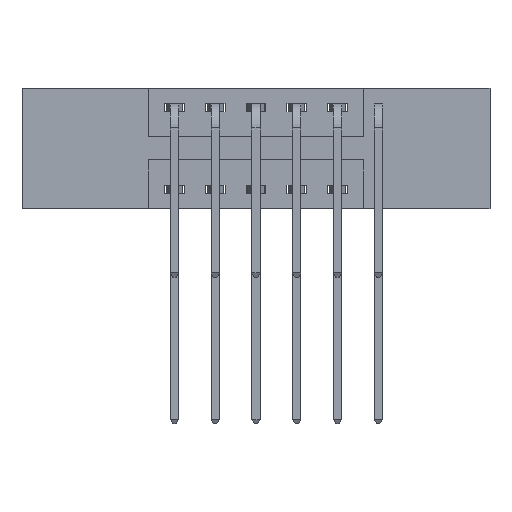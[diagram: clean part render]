
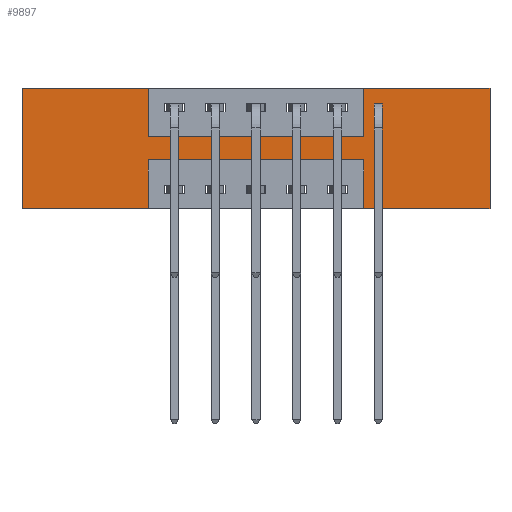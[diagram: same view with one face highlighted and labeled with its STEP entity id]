
A CAD part, front view. The second image highlights one B-rep face of the part: STEP entity #9897.
In plain terms, the highlighted planar face has unit normal (0, -1, 0).
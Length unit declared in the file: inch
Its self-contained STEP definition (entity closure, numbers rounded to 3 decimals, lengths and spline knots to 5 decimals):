
#41 = CARTESIAN_POINT ( 'NONE',  ( 1.435, 0., -0.37 ) ) ;
#46 = CARTESIAN_POINT ( 'NONE',  ( 0., 0., -0.37 ) ) ;
#98 = VECTOR ( 'NONE', #6321, 39.37008 ) ;
#140 = VERTEX_POINT ( 'NONE', #5157 ) ;
#458 = EDGE_CURVE ( 'NONE', #7896, #7610, #5863, .T. ) ;
#606 = CARTESIAN_POINT ( 'NONE',  ( 1.435, 0., 0. ) ) ;
#883 = VERTEX_POINT ( 'NONE', #3703 ) ;
#994 = CARTESIAN_POINT ( 'NONE',  ( 1.435, 0., 0. ) ) ;
#1152 = VERTEX_POINT ( 'NONE', #41 ) ;
#1199 = EDGE_CURVE ( 'NONE', #9735, #4054, #1919, .T. ) ;
#1211 = LINE ( 'NONE', #994, #6348 ) ;
#1308 = DIRECTION ( 'NONE',  ( 0., 0., 1. ) ) ;
#1459 = CARTESIAN_POINT ( 'NONE',  ( 0.3875, 0., -0.37 ) ) ;
#1533 = CARTESIAN_POINT ( 'NONE',  ( 0., 0., 0. ) ) ;
#1675 = VECTOR ( 'NONE', #2664, 39.37008 ) ;
#1687 = VECTOR ( 'NONE', #7762, 39.37008 ) ;
#1724 = EDGE_LOOP ( 'NONE', ( #9180, #6241, #3823, #4499, #4853, #9220, #1844, #4583, #4867, #7285, #4991, #7064 ) ) ;
#1844 = ORIENTED_EDGE ( 'NONE', *, *, #5600, .F. ) ;
#1856 = DIRECTION ( 'NONE',  ( 0., -1., 0. ) ) ;
#1919 = LINE ( 'NONE', #9070, #9211 ) ;
#2128 = LINE ( 'NONE', #1459, #5531 ) ;
#2365 = EDGE_CURVE ( 'NONE', #140, #2655, #6531, .T. ) ;
#2530 = VERTEX_POINT ( 'NONE', #3229 ) ;
#2655 = VERTEX_POINT ( 'NONE', #8426 ) ;
#2664 = DIRECTION ( 'NONE',  ( 0., 0., -1. ) ) ;
#2709 = CARTESIAN_POINT ( 'NONE',  ( 0., 0., 0. ) ) ;
#2813 = LINE ( 'NONE', #6730, #1675 ) ;
#3221 = CARTESIAN_POINT ( 'NONE',  ( 1.0475, 0., 0. ) ) ;
#3229 = CARTESIAN_POINT ( 'NONE',  ( 1.0475, 0., 0. ) ) ;
#3276 = CARTESIAN_POINT ( 'NONE',  ( 0., 0., 0. ) ) ;
#3323 = DIRECTION ( 'NONE',  ( 0., 0., -1. ) ) ;
#3421 = FACE_OUTER_BOUND ( 'NONE', #1724, .T. ) ;
#3545 = DIRECTION ( 'NONE',  ( 0., 0., 1. ) ) ;
#3548 = EDGE_CURVE ( 'NONE', #4054, #8910, #2813, .T. ) ;
#3703 = CARTESIAN_POINT ( 'NONE',  ( 1.0475, 0., -0.37 ) ) ;
#3823 = ORIENTED_EDGE ( 'NONE', *, *, #7267, .F. ) ;
#4054 = VERTEX_POINT ( 'NONE', #9973 ) ;
#4129 = DIRECTION ( 'NONE',  ( -1., 0., 0. ) ) ;
#4168 = DIRECTION ( 'NONE',  ( 0., 0., -1. ) ) ;
#4171 = VERTEX_POINT ( 'NONE', #9597 ) ;
#4249 = AXIS2_PLACEMENT_3D ( 'NONE', #9752, #1856, #3323 ) ;
#4404 = VECTOR ( 'NONE', #3545, 39.37008 ) ;
#4499 = ORIENTED_EDGE ( 'NONE', *, *, #7570, .F. ) ;
#4583 = ORIENTED_EDGE ( 'NONE', *, *, #4963, .F. ) ;
#4853 = ORIENTED_EDGE ( 'NONE', *, *, #9495, .F. ) ;
#4867 = ORIENTED_EDGE ( 'NONE', *, *, #3548, .F. ) ;
#4963 = EDGE_CURVE ( 'NONE', #8910, #4171, #8675, .T. ) ;
#4991 = ORIENTED_EDGE ( 'NONE', *, *, #9981, .F. ) ;
#5035 = LINE ( 'NONE', #8231, #4404 ) ;
#5108 = VECTOR ( 'NONE', #9667, 39.37008 ) ;
#5157 = CARTESIAN_POINT ( 'NONE',  ( 1.0475, 0., -0.22 ) ) ;
#5531 = VECTOR ( 'NONE', #9964, 39.37008 ) ;
#5600 = EDGE_CURVE ( 'NONE', #4171, #2530, #8314, .T. ) ;
#5735 = VECTOR ( 'NONE', #4129, 39.37008 ) ;
#5751 = LINE ( 'NONE', #2709, #7991 ) ;
#5863 = LINE ( 'NONE', #5962, #5108 ) ;
#5962 = CARTESIAN_POINT ( 'NONE',  ( 0., 0., -0.37 ) ) ;
#6241 = ORIENTED_EDGE ( 'NONE', *, *, #2365, .F. ) ;
#6321 = DIRECTION ( 'NONE',  ( -1., 0., 0. ) ) ;
#6348 = VECTOR ( 'NONE', #4168, 39.37008 ) ;
#6393 = EDGE_CURVE ( 'NONE', #2655, #7896, #2128, .T. ) ;
#6531 = LINE ( 'NONE', #9519, #5735 ) ;
#6652 = PLANE ( 'NONE',  #4249 ) ;
#6730 = CARTESIAN_POINT ( 'NONE',  ( 0.3875, 0., 0. ) ) ;
#6998 = VECTOR ( 'NONE', #9552, 39.37008 ) ;
#7064 = ORIENTED_EDGE ( 'NONE', *, *, #458, .F. ) ;
#7090 = LINE ( 'NONE', #46, #98 ) ;
#7267 = EDGE_CURVE ( 'NONE', #883, #140, #5035, .T. ) ;
#7285 = ORIENTED_EDGE ( 'NONE', *, *, #1199, .F. ) ;
#7482 = LINE ( 'NONE', #1533, #9790 ) ;
#7504 = DIRECTION ( 'NONE',  ( 1., 0., 0. ) ) ;
#7570 = EDGE_CURVE ( 'NONE', #1152, #883, #7090, .T. ) ;
#7610 = VERTEX_POINT ( 'NONE', #8118 ) ;
#7674 = EDGE_CURVE ( 'NONE', #2530, #8698, #5751, .T. ) ;
#7762 = DIRECTION ( 'NONE',  ( 1., 0., 0. ) ) ;
#7896 = VERTEX_POINT ( 'NONE', #10062 ) ;
#7910 = CARTESIAN_POINT ( 'NONE',  ( 0.3875, 0., -0.15 ) ) ;
#7991 = VECTOR ( 'NONE', #7504, 39.37008 ) ;
#8118 = CARTESIAN_POINT ( 'NONE',  ( 0., 0., -0.37 ) ) ;
#8231 = CARTESIAN_POINT ( 'NONE',  ( 1.0475, 0., -0.37 ) ) ;
#8314 = LINE ( 'NONE', #3221, #6998 ) ;
#8426 = CARTESIAN_POINT ( 'NONE',  ( 0.3875, 0., -0.22 ) ) ;
#8675 = LINE ( 'NONE', #7910, #1687 ) ;
#8698 = VERTEX_POINT ( 'NONE', #606 ) ;
#8729 = CARTESIAN_POINT ( 'NONE',  ( 0.3875, 0., -0.15 ) ) ;
#8910 = VERTEX_POINT ( 'NONE', #8729 ) ;
#9070 = CARTESIAN_POINT ( 'NONE',  ( 0., 0., 0. ) ) ;
#9180 = ORIENTED_EDGE ( 'NONE', *, *, #6393, .F. ) ;
#9211 = VECTOR ( 'NONE', #9771, 39.37008 ) ;
#9220 = ORIENTED_EDGE ( 'NONE', *, *, #7674, .F. ) ;
#9495 = EDGE_CURVE ( 'NONE', #8698, #1152, #1211, .T. ) ;
#9519 = CARTESIAN_POINT ( 'NONE',  ( 0.3875, 0., -0.22 ) ) ;
#9552 = DIRECTION ( 'NONE',  ( 0., 0., 1. ) ) ;
#9597 = CARTESIAN_POINT ( 'NONE',  ( 1.0475, 0., -0.15 ) ) ;
#9667 = DIRECTION ( 'NONE',  ( -1., 0., 0. ) ) ;
#9735 = VERTEX_POINT ( 'NONE', #3276 ) ;
#9752 = CARTESIAN_POINT ( 'NONE',  ( 0., 0., -0.37 ) ) ;
#9771 = DIRECTION ( 'NONE',  ( 1., 0., 0. ) ) ;
#9790 = VECTOR ( 'NONE', #1308, 39.37008 ) ;
#9897 = ADVANCED_FACE ( 'NONE', ( #3421 ), #6652, .T. ) ;
#9964 = DIRECTION ( 'NONE',  ( 0., 0., -1. ) ) ;
#9973 = CARTESIAN_POINT ( 'NONE',  ( 0.3875, 0., 0. ) ) ;
#9981 = EDGE_CURVE ( 'NONE', #7610, #9735, #7482, .T. ) ;
#10062 = CARTESIAN_POINT ( 'NONE',  ( 0.3875, 0., -0.37 ) ) ;
